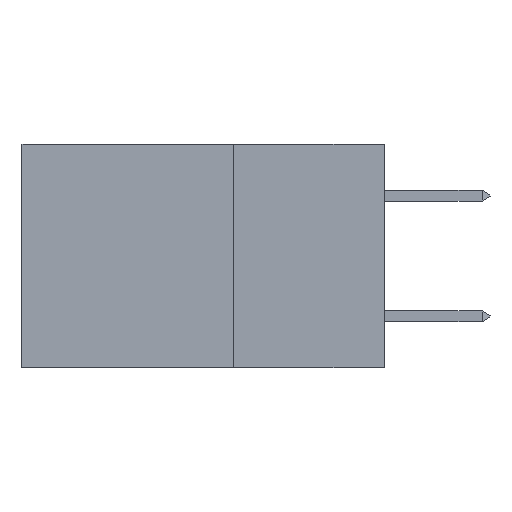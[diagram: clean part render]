
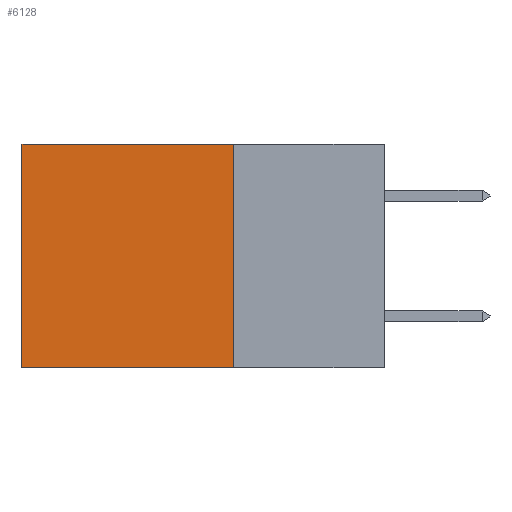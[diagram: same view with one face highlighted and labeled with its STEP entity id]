
A CAD part, left-side view. The second image highlights one B-rep face of the part: STEP entity #6128.
In plain terms, the highlighted planar face has unit normal (-1, 0, 0).
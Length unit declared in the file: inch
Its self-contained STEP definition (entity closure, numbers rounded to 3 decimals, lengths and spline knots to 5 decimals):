
#208 = DIRECTION ( 'NONE',  ( 0., 0., -1. ) ) ;
#495 = CARTESIAN_POINT ( 'NONE',  ( 0.2875, 0.6, 0. ) ) ;
#515 = VECTOR ( 'NONE', #12114, 39.37008 ) ;
#714 = VECTOR ( 'NONE', #12514, 39.37008 ) ;
#855 = CARTESIAN_POINT ( 'NONE',  ( 0.2875, 0.25, -0.37 ) ) ;
#1539 = CARTESIAN_POINT ( 'NONE',  ( 0.2875, 0.25, 0. ) ) ;
#2833 = DIRECTION ( 'NONE',  ( 1., 0., 0. ) ) ;
#3229 = EDGE_CURVE ( 'NONE', #16170, #12687, #20895, .T. ) ;
#3504 = CARTESIAN_POINT ( 'NONE',  ( 0.2875, 0.6, 0. ) ) ;
#5611 = DIRECTION ( 'NONE',  ( 0., 0., -1. ) ) ;
#6062 = CARTESIAN_POINT ( 'NONE',  ( 0.2875, 0.25, -0.37 ) ) ;
#6128 = ADVANCED_FACE ( 'NONE', ( #27472 ), #25815, .F. ) ;
#6365 = ORIENTED_EDGE ( 'NONE', *, *, #18883, .F. ) ;
#7261 = LINE ( 'NONE', #495, #16251 ) ;
#7399 = EDGE_CURVE ( 'NONE', #14376, #12687, #7261, .T. ) ;
#8221 = AXIS2_PLACEMENT_3D ( 'NONE', #23312, #2833, #5611 ) ;
#9410 = LINE ( 'NONE', #11160, #11977 ) ;
#9555 = DIRECTION ( 'NONE',  ( 0., 1., 0. ) ) ;
#11160 = CARTESIAN_POINT ( 'NONE',  ( 0.2875, 0.25, 0. ) ) ;
#11977 = VECTOR ( 'NONE', #9555, 39.37008 ) ;
#12114 = DIRECTION ( 'NONE',  ( 0., 1., 0. ) ) ;
#12514 = DIRECTION ( 'NONE',  ( 0., 0., -1. ) ) ;
#12687 = VERTEX_POINT ( 'NONE', #18016 ) ;
#14376 = VERTEX_POINT ( 'NONE', #3504 ) ;
#16170 = VERTEX_POINT ( 'NONE', #6062 ) ;
#16251 = VECTOR ( 'NONE', #208, 39.37008 ) ;
#17192 = EDGE_LOOP ( 'NONE', ( #18543, #21571, #6365, #23811 ) ) ;
#18016 = CARTESIAN_POINT ( 'NONE',  ( 0.2875, 0.6, -0.37 ) ) ;
#18540 = CARTESIAN_POINT ( 'NONE',  ( 0.2875, 0.25, 0. ) ) ;
#18543 = ORIENTED_EDGE ( 'NONE', *, *, #7399, .T. ) ;
#18883 = EDGE_CURVE ( 'NONE', #28406, #16170, #28374, .T. ) ;
#20895 = LINE ( 'NONE', #855, #515 ) ;
#21571 = ORIENTED_EDGE ( 'NONE', *, *, #3229, .F. ) ;
#22141 = EDGE_CURVE ( 'NONE', #28406, #14376, #9410, .T. ) ;
#23312 = CARTESIAN_POINT ( 'NONE',  ( 0.2875, 0.25, 0. ) ) ;
#23811 = ORIENTED_EDGE ( 'NONE', *, *, #22141, .T. ) ;
#25815 = PLANE ( 'NONE',  #8221 ) ;
#27472 = FACE_OUTER_BOUND ( 'NONE', #17192, .T. ) ;
#28374 = LINE ( 'NONE', #1539, #714 ) ;
#28406 = VERTEX_POINT ( 'NONE', #18540 ) ;
